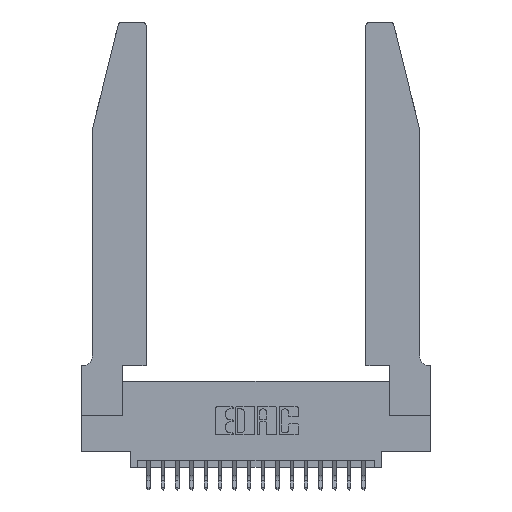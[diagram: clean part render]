
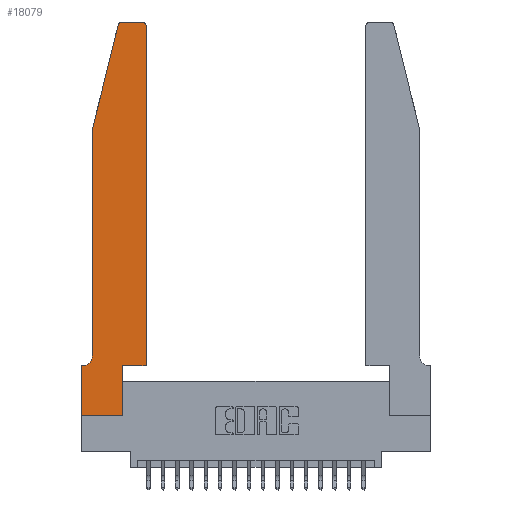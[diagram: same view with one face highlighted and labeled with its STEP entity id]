
A CAD part, top view. The second image highlights one B-rep face of the part: STEP entity #18079.
In plain terms, the highlighted planar face has unit normal (0, 0, 1).
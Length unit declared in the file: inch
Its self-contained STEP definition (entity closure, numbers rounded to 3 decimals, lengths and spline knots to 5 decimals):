
#513 = VERTEX_POINT ( 'NONE', #1627 ) ;
#895 = EDGE_CURVE ( 'NONE', #6801, #5390, #20889, .T. ) ;
#1252 = CARTESIAN_POINT ( 'NONE',  ( 0.4205, 2.75, 0.37 ) ) ;
#1382 = VERTEX_POINT ( 'NONE', #9824 ) ;
#1447 = ORIENTED_EDGE ( 'NONE', *, *, #16189, .T. ) ;
#1518 = DIRECTION ( 'NONE',  ( -0.239, -0.971, 0. ) ) ;
#1542 = ORIENTED_EDGE ( 'NONE', *, *, #8100, .T. ) ;
#1627 = CARTESIAN_POINT ( 'NONE',  ( 0.4505, 2.72, 0.37 ) ) ;
#1660 = ORIENTED_EDGE ( 'NONE', *, *, #19923, .T. ) ;
#1736 = CARTESIAN_POINT ( 'NONE',  ( 0.0055, 0.42, 0.37 ) ) ;
#2433 = CARTESIAN_POINT ( 'NONE',  ( 0., 0., 0.37 ) ) ;
#2479 = ORIENTED_EDGE ( 'NONE', *, *, #6849, .T. ) ;
#2662 = ORIENTED_EDGE ( 'NONE', *, *, #10327, .T. ) ;
#2711 = CARTESIAN_POINT ( 'NONE',  ( 0.2605, 2.75, 0.37 ) ) ;
#2942 = LINE ( 'NONE', #11421, #20167 ) ;
#3179 = ORIENTED_EDGE ( 'NONE', *, *, #19805, .T. ) ;
#3460 = DIRECTION ( 'NONE',  ( -1., 0., 0. ) ) ;
#3505 = CIRCLE ( 'NONE', #18854, 0.03 ) ;
#3831 = CIRCLE ( 'NONE', #19505, 0.03 ) ;
#3838 = VECTOR ( 'NONE', #13647, 39.37008 ) ;
#4372 = DIRECTION ( 'NONE',  ( -1., 0., 0. ) ) ;
#4402 = CARTESIAN_POINT ( 'NONE',  ( 0.4205, 2.72, 0.37 ) ) ;
#5030 = AXIS2_PLACEMENT_3D ( 'NONE', #21103, #19595, #10021 ) ;
#5390 = VERTEX_POINT ( 'NONE', #11995 ) ;
#5640 = VERTEX_POINT ( 'NONE', #12849 ) ;
#5885 = DIRECTION ( 'NONE',  ( 0., 1., 0. ) ) ;
#6060 = DIRECTION ( 'NONE',  ( 1., 0., 0. ) ) ;
#6127 = LINE ( 'NONE', #6982, #13780 ) ;
#6210 = EDGE_CURVE ( 'NONE', #18577, #5640, #10963, .T. ) ;
#6801 = VERTEX_POINT ( 'NONE', #13867 ) ;
#6849 = EDGE_CURVE ( 'NONE', #15183, #513, #9186, .T. ) ;
#6889 = CARTESIAN_POINT ( 'NONE',  ( 0.0755, 0.42, 0.37 ) ) ;
#6982 = CARTESIAN_POINT ( 'NONE',  ( 0.0755, 2., 0.37 ) ) ;
#7481 = DIRECTION ( 'NONE',  ( 0., 0., 1. ) ) ;
#8100 = EDGE_CURVE ( 'NONE', #5640, #19517, #3831, .T. ) ;
#8338 = PLANE ( 'NONE',  #5030 ) ;
#8535 = VERTEX_POINT ( 'NONE', #6889 ) ;
#8572 = DIRECTION ( 'NONE',  ( 1., 0., 0. ) ) ;
#9050 = AXIS2_PLACEMENT_3D ( 'NONE', #1736, #13285, #3460 ) ;
#9186 = LINE ( 'NONE', #17232, #17743 ) ;
#9824 = CARTESIAN_POINT ( 'NONE',  ( 0.2865, 0.35, 0.37 ) ) ;
#9953 = DIRECTION ( 'NONE',  ( 1., 0., 0. ) ) ;
#10005 = VECTOR ( 'NONE', #8572, 39.37008 ) ;
#10021 = DIRECTION ( 'NONE',  ( 1., 0., 0. ) ) ;
#10192 = CARTESIAN_POINT ( 'NONE',  ( 0.0755, 2., 0.37 ) ) ;
#10237 = EDGE_CURVE ( 'NONE', #19517, #19396, #2942, .T. ) ;
#10315 = DIRECTION ( 'NONE',  ( 0., -1., 0. ) ) ;
#10327 = EDGE_CURVE ( 'NONE', #8535, #20193, #13947, .T. ) ;
#10388 = ORIENTED_EDGE ( 'NONE', *, *, #10237, .T. ) ;
#10654 = CARTESIAN_POINT ( 'NONE',  ( 0.0055, 0.35, 0.37 ) ) ;
#10963 = LINE ( 'NONE', #2711, #15237 ) ;
#10984 = DIRECTION ( 'NONE',  ( 0., -1., 0. ) ) ;
#11155 = DIRECTION ( 'NONE',  ( -1., 0., 0. ) ) ;
#11421 = CARTESIAN_POINT ( 'NONE',  ( 0.0755, 2., 0.37 ) ) ;
#11575 = CARTESIAN_POINT ( 'NONE',  ( 0.2865, 0., 0.37 ) ) ;
#11995 = CARTESIAN_POINT ( 'NONE',  ( 0., 0., 0.37 ) ) ;
#12425 = ORIENTED_EDGE ( 'NONE', *, *, #895, .T. ) ;
#12849 = CARTESIAN_POINT ( 'NONE',  ( 0.284, 2.75, 0.37 ) ) ;
#12959 = VECTOR ( 'NONE', #10984, 39.37008 ) ;
#13285 = DIRECTION ( 'NONE',  ( 0., 0., -1. ) ) ;
#13395 = EDGE_LOOP ( 'NONE', ( #17908, #1542, #10388, #18903, #2662, #3179, #12425, #13447, #1447, #1660, #2479, #20473 ) ) ;
#13447 = ORIENTED_EDGE ( 'NONE', *, *, #16794, .T. ) ;
#13647 = DIRECTION ( 'NONE',  ( 0., 1., 0. ) ) ;
#13780 = VECTOR ( 'NONE', #10315, 39.37008 ) ;
#13867 = CARTESIAN_POINT ( 'NONE',  ( 0., 0.35, 0.37 ) ) ;
#13899 = VECTOR ( 'NONE', #11155, 39.37008 ) ;
#13947 = CIRCLE ( 'NONE', #9050, 0.07 ) ;
#14278 = LINE ( 'NONE', #19744, #10005 ) ;
#14390 = VERTEX_POINT ( 'NONE', #11575 ) ;
#14396 = LINE ( 'NONE', #20762, #13899 ) ;
#15183 = VERTEX_POINT ( 'NONE', #17597 ) ;
#15237 = VECTOR ( 'NONE', #4372, 39.37008 ) ;
#15638 = VECTOR ( 'NONE', #9953, 39.37008 ) ;
#15782 = DIRECTION ( 'NONE',  ( 0., 0., 1. ) ) ;
#16189 = EDGE_CURVE ( 'NONE', #14390, #1382, #20998, .T. ) ;
#16786 = CARTESIAN_POINT ( 'NONE',  ( 0.25487, 2.72718, 0.37 ) ) ;
#16794 = EDGE_CURVE ( 'NONE', #5390, #14390, #14278, .T. ) ;
#16818 = EDGE_CURVE ( 'NONE', #19396, #8535, #6127, .T. ) ;
#17185 = CARTESIAN_POINT ( 'NONE',  ( 0.284, 2.72, 0.37 ) ) ;
#17232 = CARTESIAN_POINT ( 'NONE',  ( 0.4505, 0.35, 0.37 ) ) ;
#17597 = CARTESIAN_POINT ( 'NONE',  ( 0.4505, 0.35, 0.37 ) ) ;
#17743 = VECTOR ( 'NONE', #5885, 39.37008 ) ;
#17853 = EDGE_CURVE ( 'NONE', #513, #18577, #3505, .T. ) ;
#17908 = ORIENTED_EDGE ( 'NONE', *, *, #6210, .T. ) ;
#17955 = CARTESIAN_POINT ( 'NONE',  ( 0.4505, 0.35, 0.37 ) ) ;
#18079 = ADVANCED_FACE ( 'NONE', ( #19939 ), #8338, .T. ) ;
#18389 = CARTESIAN_POINT ( 'NONE',  ( 0.2865, 0.35, 0.37 ) ) ;
#18577 = VERTEX_POINT ( 'NONE', #1252 ) ;
#18780 = DIRECTION ( 'NONE',  ( 1., 0., 0. ) ) ;
#18854 = AXIS2_PLACEMENT_3D ( 'NONE', #4402, #15782, #6060 ) ;
#18903 = ORIENTED_EDGE ( 'NONE', *, *, #16818, .T. ) ;
#19396 = VERTEX_POINT ( 'NONE', #10192 ) ;
#19505 = AXIS2_PLACEMENT_3D ( 'NONE', #17185, #7481, #18780 ) ;
#19517 = VERTEX_POINT ( 'NONE', #16786 ) ;
#19595 = DIRECTION ( 'NONE',  ( 0., 0., 1. ) ) ;
#19744 = CARTESIAN_POINT ( 'NONE',  ( 0., 0., 0.37 ) ) ;
#19805 = EDGE_CURVE ( 'NONE', #20193, #6801, #14396, .T. ) ;
#19923 = EDGE_CURVE ( 'NONE', #1382, #15183, #20355, .T. ) ;
#19939 = FACE_OUTER_BOUND ( 'NONE', #13395, .T. ) ;
#20167 = VECTOR ( 'NONE', #1518, 39.37008 ) ;
#20193 = VERTEX_POINT ( 'NONE', #10654 ) ;
#20355 = LINE ( 'NONE', #17955, #15638 ) ;
#20473 = ORIENTED_EDGE ( 'NONE', *, *, #17853, .T. ) ;
#20762 = CARTESIAN_POINT ( 'NONE',  ( 0.0755, 0.35, 0.37 ) ) ;
#20889 = LINE ( 'NONE', #2433, #12959 ) ;
#20998 = LINE ( 'NONE', #18389, #3838 ) ;
#21103 = CARTESIAN_POINT ( 'NONE',  ( 0., 0.35, 0.37 ) ) ;
